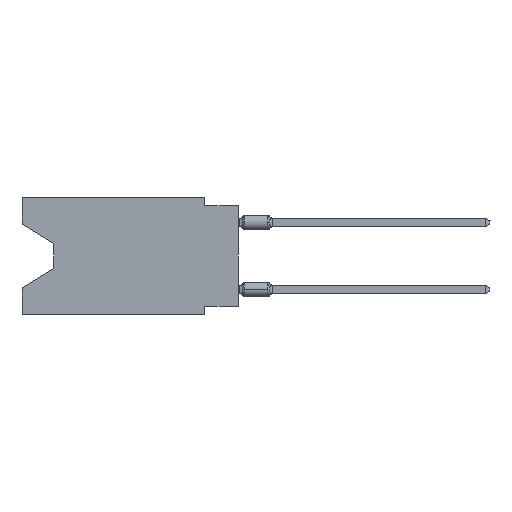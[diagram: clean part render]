
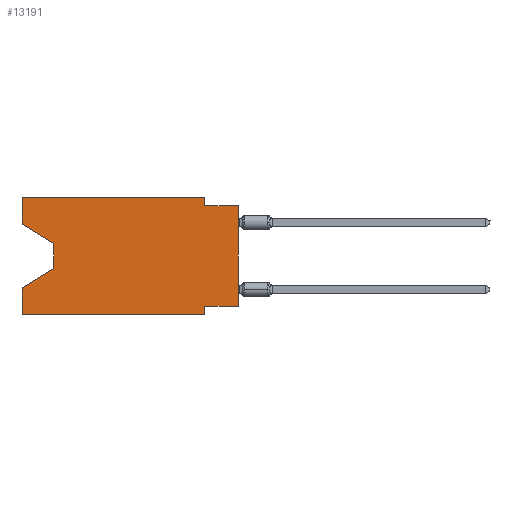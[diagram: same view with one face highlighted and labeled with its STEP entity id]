
A CAD part, left-side view. The second image highlights one B-rep face of the part: STEP entity #13191.
In plain terms, the highlighted planar face has unit normal (-1, 0, 0).
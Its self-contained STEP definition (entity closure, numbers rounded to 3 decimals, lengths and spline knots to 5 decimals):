
#1990 = LINE ( 'NONE', #17329, #48547 ) ;
#2724 = EDGE_CURVE ( 'NONE', #3318, #63408, #35364, .T. ) ;
#2960 = ORIENTED_EDGE ( 'NONE', *, *, #19509, .T. ) ;
#3197 = DIRECTION ( 'NONE',  ( 0., 0., 1. ) ) ;
#3318 = VERTEX_POINT ( 'NONE', #59085 ) ;
#3751 = LINE ( 'NONE', #10071, #62328 ) ;
#4163 = CARTESIAN_POINT ( 'NONE',  ( 0., 0.645, 0. ) ) ;
#4233 = DIRECTION ( 'NONE',  ( 0., 0., 1. ) ) ;
#5163 = LINE ( 'NONE', #33885, #46686 ) ;
#8246 = EDGE_CURVE ( 'NONE', #45360, #45026, #8905, .T. ) ;
#8351 = EDGE_CURVE ( 'NONE', #36773, #18589, #67376, .T. ) ;
#8905 = LINE ( 'NONE', #15593, #21483 ) ;
#9576 = EDGE_CURVE ( 'NONE', #45026, #59568, #5163, .T. ) ;
#10071 = CARTESIAN_POINT ( 'NONE',  ( 0., 0.645, -0.08025 ) ) ;
#11103 = DIRECTION ( 'NONE',  ( 0., 0., -1. ) ) ;
#11341 = ORIENTED_EDGE ( 'NONE', *, *, #63820, .T. ) ;
#11510 = VERTEX_POINT ( 'NONE', #49212 ) ;
#12011 = AXIS2_PLACEMENT_3D ( 'NONE', #26232, #51093, #26596 ) ;
#12562 = ORIENTED_EDGE ( 'NONE', *, *, #2724, .F. ) ;
#12931 = EDGE_CURVE ( 'NONE', #11510, #18658, #56495, .T. ) ;
#13191 = ADVANCED_FACE ( 'NONE', ( #56675 ), #15017, .F. ) ;
#13955 = VERTEX_POINT ( 'NONE', #70679 ) ;
#15017 = PLANE ( 'NONE',  #12011 ) ;
#15593 = CARTESIAN_POINT ( 'NONE',  ( 0., 0., -0.325 ) ) ;
#16980 = DIRECTION ( 'NONE',  ( 0., 0., -1. ) ) ;
#17329 = CARTESIAN_POINT ( 'NONE',  ( 0., 0.55, -0.212 ) ) ;
#18429 = DIRECTION ( 'NONE',  ( 0., 0.855, -0.519 ) ) ;
#18589 = VERTEX_POINT ( 'NONE', #64081 ) ;
#18658 = VERTEX_POINT ( 'NONE', #32750 ) ;
#19509 = EDGE_CURVE ( 'NONE', #3318, #36773, #3751, .T. ) ;
#21483 = VECTOR ( 'NONE', #55503, 39.37008 ) ;
#21719 = DIRECTION ( 'NONE',  ( 0., -1., 0. ) ) ;
#23796 = CARTESIAN_POINT ( 'NONE',  ( 0., 0.645, 0. ) ) ;
#25590 = LINE ( 'NONE', #48360, #47855 ) ;
#25864 = ORIENTED_EDGE ( 'NONE', *, *, #8246, .F. ) ;
#26232 = CARTESIAN_POINT ( 'NONE',  ( 0., 0.645, 0. ) ) ;
#26270 = ORIENTED_EDGE ( 'NONE', *, *, #32886, .F. ) ;
#26596 = DIRECTION ( 'NONE',  ( 0., 0., -1. ) ) ;
#27222 = DIRECTION ( 'NONE',  ( 0., -0.855, -0.519 ) ) ;
#27915 = DIRECTION ( 'NONE',  ( 0., 0., -1. ) ) ;
#32750 = CARTESIAN_POINT ( 'NONE',  ( 0., 0.1, -0.025 ) ) ;
#32886 = EDGE_CURVE ( 'NONE', #63408, #11510, #37758, .T. ) ;
#32961 = CARTESIAN_POINT ( 'NONE',  ( 0., 0., 0. ) ) ;
#33281 = ORIENTED_EDGE ( 'NONE', *, *, #63263, .F. ) ;
#33657 = LINE ( 'NONE', #44829, #59121 ) ;
#33885 = CARTESIAN_POINT ( 'NONE',  ( 0., 0.1, -0.35 ) ) ;
#34507 = CARTESIAN_POINT ( 'NONE',  ( 0., 0.1, 0. ) ) ;
#35364 = LINE ( 'NONE', #23796, #53601 ) ;
#36773 = VERTEX_POINT ( 'NONE', #67413 ) ;
#37758 = LINE ( 'NONE', #4163, #48081 ) ;
#38496 = DIRECTION ( 'NONE',  ( 0., -1., 0. ) ) ;
#38657 = CARTESIAN_POINT ( 'NONE',  ( 0., 0.645, 0. ) ) ;
#38970 = VERTEX_POINT ( 'NONE', #55093 ) ;
#39500 = CARTESIAN_POINT ( 'NONE',  ( 0., 0.645, -0.35 ) ) ;
#39834 = CARTESIAN_POINT ( 'NONE',  ( 0., 0.55, -0.138 ) ) ;
#39868 = VERTEX_POINT ( 'NONE', #39500 ) ;
#42138 = ORIENTED_EDGE ( 'NONE', *, *, #9576, .F. ) ;
#44105 = LINE ( 'NONE', #55275, #61859 ) ;
#44478 = EDGE_LOOP ( 'NONE', ( #2960, #61290, #71524, #60836, #45790, #42138, #25864, #11341, #33281, #59397, #26270, #12562 ) ) ;
#44829 = CARTESIAN_POINT ( 'NONE',  ( 0., 0.645, -0.35 ) ) ;
#45026 = VERTEX_POINT ( 'NONE', #69522 ) ;
#45262 = VECTOR ( 'NONE', #4233, 39.37008 ) ;
#45360 = VERTEX_POINT ( 'NONE', #69781 ) ;
#45790 = ORIENTED_EDGE ( 'NONE', *, *, #57662, .T. ) ;
#46686 = VECTOR ( 'NONE', #27915, 39.37008 ) ;
#47855 = VECTOR ( 'NONE', #3197, 39.37008 ) ;
#48081 = VECTOR ( 'NONE', #38496, 39.37008 ) ;
#48360 = CARTESIAN_POINT ( 'NONE',  ( 0., 0.645, 0. ) ) ;
#48547 = VECTOR ( 'NONE', #18429, 39.37008 ) ;
#49212 = CARTESIAN_POINT ( 'NONE',  ( 0., 0.1, 0. ) ) ;
#49682 = DIRECTION ( 'NONE',  ( 0., -1., 0. ) ) ;
#49868 = EDGE_CURVE ( 'NONE', #39868, #13955, #25590, .T. ) ;
#51093 = DIRECTION ( 'NONE',  ( 1., 0., 0. ) ) ;
#52426 = CARTESIAN_POINT ( 'NONE',  ( 0., 0.1, -0.35 ) ) ;
#53601 = VECTOR ( 'NONE', #69247, 39.37008 ) ;
#54852 = VECTOR ( 'NONE', #11103, 39.37008 ) ;
#55093 = CARTESIAN_POINT ( 'NONE',  ( 0., 0., -0.025 ) ) ;
#55275 = CARTESIAN_POINT ( 'NONE',  ( 0., 0., -0.025 ) ) ;
#55503 = DIRECTION ( 'NONE',  ( 0., 1., 0. ) ) ;
#56495 = LINE ( 'NONE', #34507, #64389 ) ;
#56675 = FACE_OUTER_BOUND ( 'NONE', #44478, .T. ) ;
#57662 = EDGE_CURVE ( 'NONE', #39868, #59568, #33657, .T. ) ;
#58676 = EDGE_CURVE ( 'NONE', #18589, #13955, #1990, .T. ) ;
#59085 = CARTESIAN_POINT ( 'NONE',  ( 0., 0.645, -0.08025 ) ) ;
#59121 = VECTOR ( 'NONE', #21719, 39.37008 ) ;
#59397 = ORIENTED_EDGE ( 'NONE', *, *, #12931, .F. ) ;
#59568 = VERTEX_POINT ( 'NONE', #52426 ) ;
#60836 = ORIENTED_EDGE ( 'NONE', *, *, #49868, .F. ) ;
#61290 = ORIENTED_EDGE ( 'NONE', *, *, #8351, .T. ) ;
#61859 = VECTOR ( 'NONE', #49682, 39.37008 ) ;
#62328 = VECTOR ( 'NONE', #27222, 39.37008 ) ;
#63263 = EDGE_CURVE ( 'NONE', #18658, #38970, #44105, .T. ) ;
#63408 = VERTEX_POINT ( 'NONE', #38657 ) ;
#63820 = EDGE_CURVE ( 'NONE', #45360, #38970, #66116, .T. ) ;
#64081 = CARTESIAN_POINT ( 'NONE',  ( 0., 0.55, -0.212 ) ) ;
#64389 = VECTOR ( 'NONE', #16980, 39.37008 ) ;
#66116 = LINE ( 'NONE', #32961, #45262 ) ;
#67376 = LINE ( 'NONE', #39834, #54852 ) ;
#67413 = CARTESIAN_POINT ( 'NONE',  ( 0., 0.55, -0.138 ) ) ;
#69247 = DIRECTION ( 'NONE',  ( 0., 0., 1. ) ) ;
#69522 = CARTESIAN_POINT ( 'NONE',  ( 0., 0.1, -0.325 ) ) ;
#69781 = CARTESIAN_POINT ( 'NONE',  ( 0., 0., -0.325 ) ) ;
#70679 = CARTESIAN_POINT ( 'NONE',  ( 0., 0.645, -0.26975 ) ) ;
#71524 = ORIENTED_EDGE ( 'NONE', *, *, #58676, .T. ) ;
